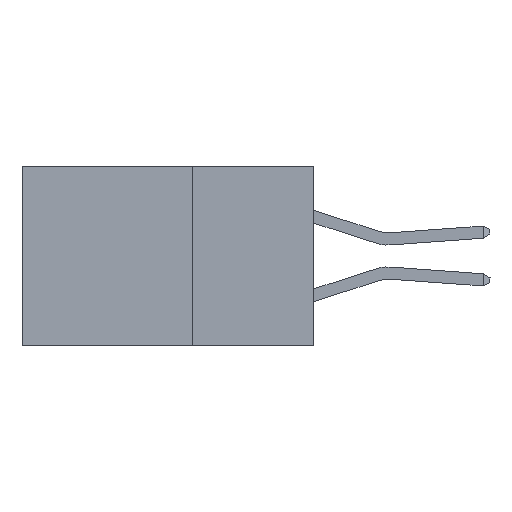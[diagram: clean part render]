
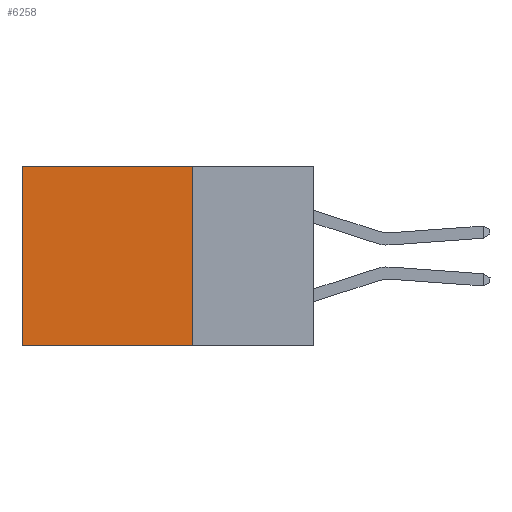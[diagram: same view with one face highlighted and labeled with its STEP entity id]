
A CAD part, left-side view. The second image highlights one B-rep face of the part: STEP entity #6258.
In plain terms, the highlighted planar face has unit normal (-1, 0, 0).
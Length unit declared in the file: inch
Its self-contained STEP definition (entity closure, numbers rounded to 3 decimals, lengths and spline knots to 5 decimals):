
#428 = CARTESIAN_POINT ( 'NONE',  ( 0.2875, 0.6, -0.37 ) ) ;
#863 = EDGE_CURVE ( 'NONE', #8324, #23977, #8632, .T. ) ;
#2206 = ORIENTED_EDGE ( 'NONE', *, *, #9118, .T. ) ;
#2694 = CARTESIAN_POINT ( 'NONE',  ( 0.2875, 0.6, 0. ) ) ;
#2983 = EDGE_CURVE ( 'NONE', #22169, #23977, #23550, .T. ) ;
#3091 = ORIENTED_EDGE ( 'NONE', *, *, #2983, .F. ) ;
#3860 = CARTESIAN_POINT ( 'NONE',  ( 0.2875, 0.25, 0. ) ) ;
#4216 = CARTESIAN_POINT ( 'NONE',  ( 0.2875, 0.25, 0. ) ) ;
#5912 = CARTESIAN_POINT ( 'NONE',  ( 0.2875, 0.25, -0.37 ) ) ;
#6258 = ADVANCED_FACE ( 'NONE', ( #9415 ), #22717, .F. ) ;
#6442 = ORIENTED_EDGE ( 'NONE', *, *, #863, .T. ) ;
#7599 = DIRECTION ( 'NONE',  ( 0., 0., -1. ) ) ;
#8095 = VECTOR ( 'NONE', #17216, 39.37008 ) ;
#8324 = VERTEX_POINT ( 'NONE', #10397 ) ;
#8632 = LINE ( 'NONE', #2694, #13062 ) ;
#8990 = VECTOR ( 'NONE', #11591, 39.37008 ) ;
#9118 = EDGE_CURVE ( 'NONE', #23021, #8324, #17150, .T. ) ;
#9415 = FACE_OUTER_BOUND ( 'NONE', #19447, .T. ) ;
#9581 = ORIENTED_EDGE ( 'NONE', *, *, #12709, .F. ) ;
#10397 = CARTESIAN_POINT ( 'NONE',  ( 0.2875, 0.6, 0. ) ) ;
#11591 = DIRECTION ( 'NONE',  ( 0., 0., -1. ) ) ;
#12708 = CARTESIAN_POINT ( 'NONE',  ( 0.2875, 0.25, -0.37 ) ) ;
#12709 = EDGE_CURVE ( 'NONE', #23021, #22169, #24136, .T. ) ;
#13062 = VECTOR ( 'NONE', #23537, 39.37008 ) ;
#13415 = DIRECTION ( 'NONE',  ( 1., 0., 0. ) ) ;
#15650 = VECTOR ( 'NONE', #22230, 39.37008 ) ;
#16599 = CARTESIAN_POINT ( 'NONE',  ( 0.2875, 0.25, 0. ) ) ;
#17150 = LINE ( 'NONE', #24387, #15650 ) ;
#17216 = DIRECTION ( 'NONE',  ( 0., 1., 0. ) ) ;
#17671 = AXIS2_PLACEMENT_3D ( 'NONE', #3860, #13415, #7599 ) ;
#19447 = EDGE_LOOP ( 'NONE', ( #6442, #3091, #9581, #2206 ) ) ;
#22169 = VERTEX_POINT ( 'NONE', #12708 ) ;
#22230 = DIRECTION ( 'NONE',  ( 0., 1., 0. ) ) ;
#22717 = PLANE ( 'NONE',  #17671 ) ;
#23021 = VERTEX_POINT ( 'NONE', #16599 ) ;
#23537 = DIRECTION ( 'NONE',  ( 0., 0., -1. ) ) ;
#23550 = LINE ( 'NONE', #5912, #8095 ) ;
#23977 = VERTEX_POINT ( 'NONE', #428 ) ;
#24136 = LINE ( 'NONE', #4216, #8990 ) ;
#24387 = CARTESIAN_POINT ( 'NONE',  ( 0.2875, 0.25, 0. ) ) ;
